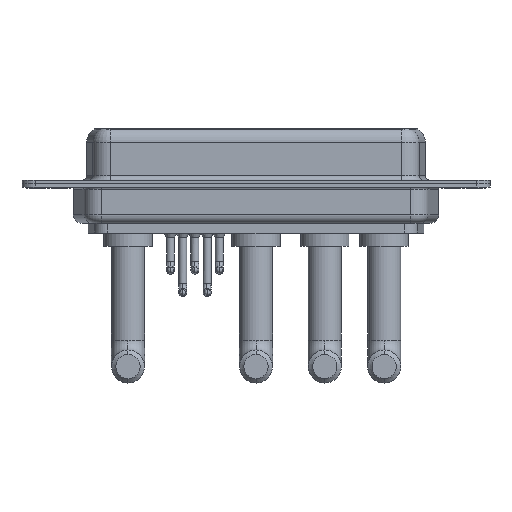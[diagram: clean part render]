
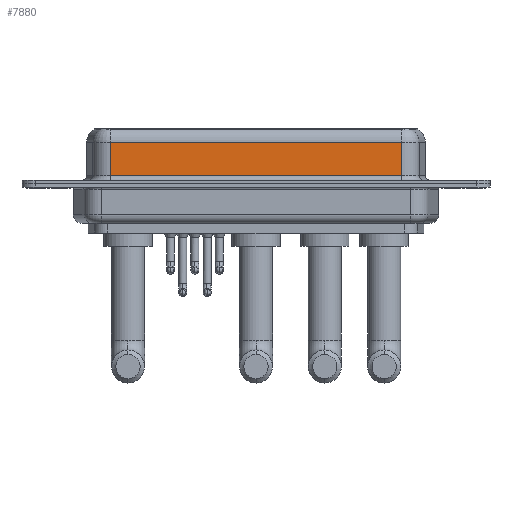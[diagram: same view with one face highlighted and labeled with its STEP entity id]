
A CAD part, front view. The second image highlights one B-rep face of the part: STEP entity #7880.
In plain terms, the highlighted planar face has unit normal (0, -1, 0).
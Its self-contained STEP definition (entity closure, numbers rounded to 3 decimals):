
#430 = LINE ( 'NONE', #11234, #445 ) ;
#445 = VECTOR ( 'NONE', #11312, 1000. ) ;
#1197 = CARTESIAN_POINT ( 'NONE',  ( 40.037, -3.95, 4.65 ) ) ;
#1437 = FACE_OUTER_BOUND ( 'NONE', #3706, .T. ) ;
#1710 = VERTEX_POINT ( 'NONE', #4193 ) ;
#1944 = DIRECTION ( 'NONE',  ( 0., 0., -1. ) ) ;
#1951 = DIRECTION ( 'NONE',  ( -1., 0., 0. ) ) ;
#2500 = ORIENTED_EDGE ( 'NONE', *, *, #13465, .T. ) ;
#3706 = EDGE_LOOP ( 'NONE', ( #8226, #2500, #10682, #14396 ) ) ;
#4193 = CARTESIAN_POINT ( 'NONE',  ( 7.013, -3.95, 0.9 ) ) ;
#4332 = VERTEX_POINT ( 'NONE', #7949 ) ;
#4594 = CARTESIAN_POINT ( 'NONE',  ( 40.037, -3.95, 6.4 ) ) ;
#5443 = VECTOR ( 'NONE', #12928, 1000. ) ;
#5671 = LINE ( 'NONE', #10581, #5443 ) ;
#6222 = PLANE ( 'NONE',  #8980 ) ;
#6267 = EDGE_CURVE ( 'NONE', #13087, #1710, #5671, .T. ) ;
#6806 = CARTESIAN_POINT ( 'NONE',  ( 40.037, -3.95, 4.65 ) ) ;
#7347 = VECTOR ( 'NONE', #1951, 1000. ) ;
#7399 = EDGE_CURVE ( 'NONE', #1710, #4332, #430, .T. ) ;
#7831 = VERTEX_POINT ( 'NONE', #1197 ) ;
#7880 = ADVANCED_FACE ( 'NONE', ( #1437 ), #6222, .F. ) ;
#7949 = CARTESIAN_POINT ( 'NONE',  ( 40.037, -3.95, 0.9 ) ) ;
#8226 = ORIENTED_EDGE ( 'NONE', *, *, #11660, .F. ) ;
#8939 = CARTESIAN_POINT ( 'NONE',  ( 7.013, -3.95, 4.65 ) ) ;
#8980 = AXIS2_PLACEMENT_3D ( 'NONE', #11915, #14432, #14506 ) ;
#9577 = VECTOR ( 'NONE', #1944, 1000. ) ;
#10581 = CARTESIAN_POINT ( 'NONE',  ( 7.013, -3.95, 6.4 ) ) ;
#10682 = ORIENTED_EDGE ( 'NONE', *, *, #6267, .T. ) ;
#11234 = CARTESIAN_POINT ( 'NONE',  ( 40.037, -3.95, 0.9 ) ) ;
#11312 = DIRECTION ( 'NONE',  ( 1., 0., 0. ) ) ;
#11421 = LINE ( 'NONE', #6806, #7347 ) ;
#11660 = EDGE_CURVE ( 'NONE', #7831, #4332, #13838, .T. ) ;
#11915 = CARTESIAN_POINT ( 'NONE',  ( 40.037, -3.95, 6.4 ) ) ;
#12928 = DIRECTION ( 'NONE',  ( 0., 0., -1. ) ) ;
#13087 = VERTEX_POINT ( 'NONE', #8939 ) ;
#13465 = EDGE_CURVE ( 'NONE', #7831, #13087, #11421, .T. ) ;
#13838 = LINE ( 'NONE', #4594, #9577 ) ;
#14396 = ORIENTED_EDGE ( 'NONE', *, *, #7399, .T. ) ;
#14432 = DIRECTION ( 'NONE',  ( 0., 1., 0. ) ) ;
#14506 = DIRECTION ( 'NONE',  ( 0., 0., 1. ) ) ;
